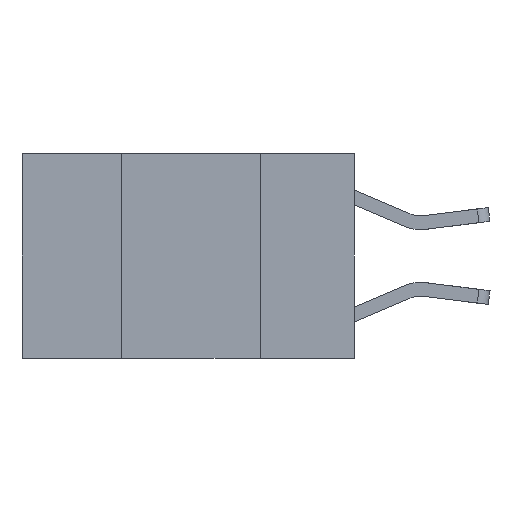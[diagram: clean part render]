
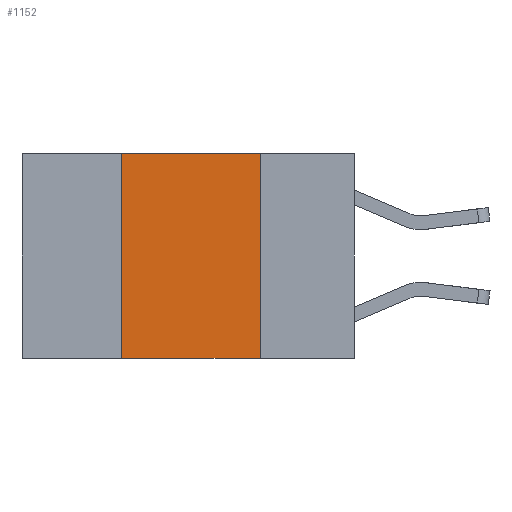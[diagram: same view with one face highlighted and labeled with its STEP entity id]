
A CAD part, left-side view. The second image highlights one B-rep face of the part: STEP entity #1152.
In plain terms, the highlighted planar face has unit normal (-1, 0, 0).
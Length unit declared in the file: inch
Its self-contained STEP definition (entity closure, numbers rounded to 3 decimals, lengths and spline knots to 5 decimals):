
#23 = AXIS2_PLACEMENT_3D ( 'NONE', #8872, #7091, #7341 ) ;
#268 = VECTOR ( 'NONE', #1336, 39.37008 ) ;
#1152 = ADVANCED_FACE ( 'NONE', ( #7825 ), #5239, .F. ) ;
#1336 = DIRECTION ( 'NONE',  ( 0., -1., 0. ) ) ;
#1624 = LINE ( 'NONE', #2255, #5251 ) ;
#1785 = EDGE_CURVE ( 'NONE', #2671, #2581, #6254, .T. ) ;
#2255 = CARTESIAN_POINT ( 'NONE',  ( 0., 0.6, 0. ) ) ;
#2581 = VERTEX_POINT ( 'NONE', #3154 ) ;
#2671 = VERTEX_POINT ( 'NONE', #5348 ) ;
#3006 = DIRECTION ( 'NONE',  ( 0., -1., 0. ) ) ;
#3154 = CARTESIAN_POINT ( 'NONE',  ( 0., 0.17, -0.37 ) ) ;
#3214 = VECTOR ( 'NONE', #6221, 39.37008 ) ;
#3259 = DIRECTION ( 'NONE',  ( 0., 0., 1. ) ) ;
#3520 = VERTEX_POINT ( 'NONE', #8709 ) ;
#3608 = VERTEX_POINT ( 'NONE', #6256 ) ;
#4167 = EDGE_LOOP ( 'NONE', ( #7123, #6603, #8002, #7814 ) ) ;
#4737 = CARTESIAN_POINT ( 'NONE',  ( 0., 0.42, 0. ) ) ;
#4883 = EDGE_CURVE ( 'NONE', #2671, #3608, #5608, .T. ) ;
#5239 = PLANE ( 'NONE',  #23 ) ;
#5251 = VECTOR ( 'NONE', #3006, 39.37008 ) ;
#5325 = EDGE_CURVE ( 'NONE', #3520, #2581, #8897, .T. ) ;
#5348 = CARTESIAN_POINT ( 'NONE',  ( 0., 0.42, -0.37 ) ) ;
#5518 = EDGE_CURVE ( 'NONE', #3608, #3520, #1624, .T. ) ;
#5608 = LINE ( 'NONE', #4737, #7274 ) ;
#6221 = DIRECTION ( 'NONE',  ( 0., 0., -1. ) ) ;
#6254 = LINE ( 'NONE', #7027, #268 ) ;
#6256 = CARTESIAN_POINT ( 'NONE',  ( 0., 0.42, 0. ) ) ;
#6603 = ORIENTED_EDGE ( 'NONE', *, *, #5518, .F. ) ;
#7027 = CARTESIAN_POINT ( 'NONE',  ( 0., 0.6, -0.37 ) ) ;
#7091 = DIRECTION ( 'NONE',  ( 1., 0., 0. ) ) ;
#7123 = ORIENTED_EDGE ( 'NONE', *, *, #5325, .F. ) ;
#7274 = VECTOR ( 'NONE', #3259, 39.37008 ) ;
#7341 = DIRECTION ( 'NONE',  ( 0., 0., -1. ) ) ;
#7814 = ORIENTED_EDGE ( 'NONE', *, *, #1785, .T. ) ;
#7825 = FACE_OUTER_BOUND ( 'NONE', #4167, .T. ) ;
#8002 = ORIENTED_EDGE ( 'NONE', *, *, #4883, .F. ) ;
#8362 = CARTESIAN_POINT ( 'NONE',  ( 0., 0.17, 0. ) ) ;
#8709 = CARTESIAN_POINT ( 'NONE',  ( 0., 0.17, 0. ) ) ;
#8872 = CARTESIAN_POINT ( 'NONE',  ( 0., 0.6, 0. ) ) ;
#8897 = LINE ( 'NONE', #8362, #3214 ) ;
